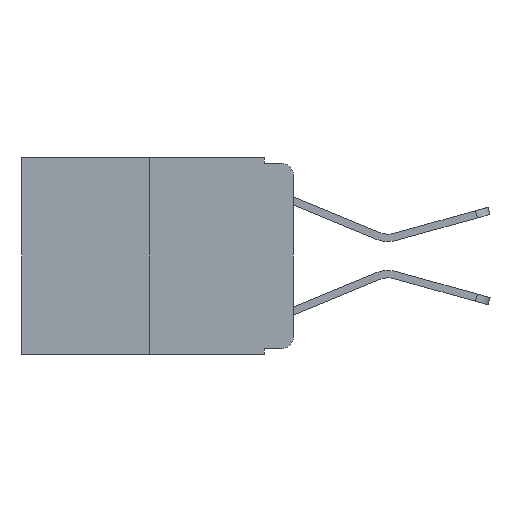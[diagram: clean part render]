
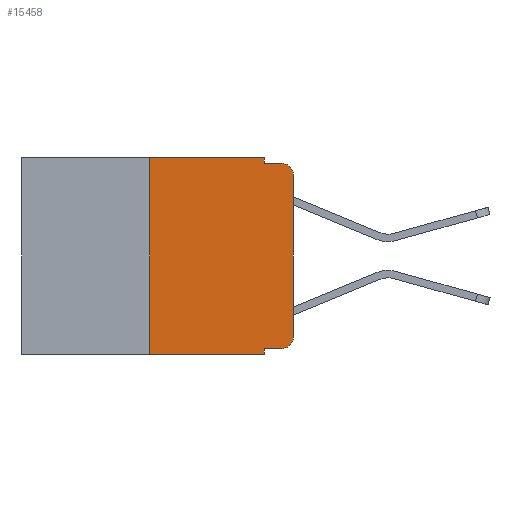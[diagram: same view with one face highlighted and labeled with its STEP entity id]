
A CAD part, left-side view. The second image highlights one B-rep face of the part: STEP entity #15458.
In plain terms, the highlighted planar face has unit normal (-1, 0, 0).
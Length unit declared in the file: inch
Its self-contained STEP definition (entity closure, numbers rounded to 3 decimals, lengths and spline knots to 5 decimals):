
#88 = CARTESIAN_POINT ( 'NONE',  ( 0., 0.051, -0.333 ) ) ;
#329 = CARTESIAN_POINT ( 'NONE',  ( 0., 0.051, -0.343 ) ) ;
#395 = FACE_OUTER_BOUND ( 'NONE', #11615, .T. ) ;
#422 = EDGE_CURVE ( 'NONE', #13965, #13686, #7644, .T. ) ;
#503 = DIRECTION ( 'NONE',  ( 0., 0., -1. ) ) ;
#634 = CARTESIAN_POINT ( 'NONE',  ( 0., 0.02, -0.03 ) ) ;
#659 = DIRECTION ( 'NONE',  ( 1., 0., 0. ) ) ;
#1108 = LINE ( 'NONE', #88, #8087 ) ;
#1526 = EDGE_CURVE ( 'NONE', #9423, #16759, #16364, .T. ) ;
#2062 = EDGE_CURVE ( 'NONE', #16759, #19306, #13859, .T. ) ;
#2522 = DIRECTION ( 'NONE',  ( 0., 0., -1. ) ) ;
#2666 = CARTESIAN_POINT ( 'NONE',  ( 0., 0.051, 0. ) ) ;
#3012 = EDGE_CURVE ( 'NONE', #3076, #13375, #11071, .T. ) ;
#3076 = VERTEX_POINT ( 'NONE', #5840 ) ;
#3400 = ORIENTED_EDGE ( 'NONE', *, *, #2062, .T. ) ;
#3526 = DIRECTION ( 'NONE',  ( 0., 0., 1. ) ) ;
#3726 = CARTESIAN_POINT ( 'NONE',  ( 0., 0., -0.313 ) ) ;
#3765 = CARTESIAN_POINT ( 'NONE',  ( 0., 0.25, 0. ) ) ;
#3791 = VECTOR ( 'NONE', #12204, 39.37008 ) ;
#4184 = VERTEX_POINT ( 'NONE', #16595 ) ;
#4256 = VERTEX_POINT ( 'NONE', #19798 ) ;
#4436 = CARTESIAN_POINT ( 'NONE',  ( 0., 0.473, -0.343 ) ) ;
#4549 = ORIENTED_EDGE ( 'NONE', *, *, #18521, .T. ) ;
#4565 = VECTOR ( 'NONE', #5202, 39.37008 ) ;
#4769 = LINE ( 'NONE', #18748, #3791 ) ;
#5177 = LINE ( 'NONE', #3765, #5943 ) ;
#5202 = DIRECTION ( 'NONE',  ( 0., -1., 0. ) ) ;
#5239 = PLANE ( 'NONE',  #6532 ) ;
#5347 = AXIS2_PLACEMENT_3D ( 'NONE', #20243, #10713, #20041 ) ;
#5450 = CARTESIAN_POINT ( 'NONE',  ( 0., 0.473, 0. ) ) ;
#5803 = CARTESIAN_POINT ( 'NONE',  ( 0., 0.051, -0.01 ) ) ;
#5840 = CARTESIAN_POINT ( 'NONE',  ( 0., 0.051, -0.333 ) ) ;
#5873 = VECTOR ( 'NONE', #3526, 39.37008 ) ;
#5907 = VECTOR ( 'NONE', #10166, 39.37008 ) ;
#5943 = VECTOR ( 'NONE', #16184, 39.37008 ) ;
#6349 = CARTESIAN_POINT ( 'NONE',  ( 0., 0.02, -0.01 ) ) ;
#6532 = AXIS2_PLACEMENT_3D ( 'NONE', #5450, #659, #6918 ) ;
#6845 = CARTESIAN_POINT ( 'NONE',  ( 0., 0.25, -0.343 ) ) ;
#6918 = DIRECTION ( 'NONE',  ( 0., 0., -1. ) ) ;
#7361 = LINE ( 'NONE', #4436, #14597 ) ;
#7644 = LINE ( 'NONE', #14907, #5907 ) ;
#7840 = VECTOR ( 'NONE', #2522, 39.37008 ) ;
#7985 = ORIENTED_EDGE ( 'NONE', *, *, #3012, .F. ) ;
#8087 = VECTOR ( 'NONE', #8300, 39.37008 ) ;
#8300 = DIRECTION ( 'NONE',  ( 0., -1., 0. ) ) ;
#8839 = CARTESIAN_POINT ( 'NONE',  ( 0., 0.473, 0. ) ) ;
#9423 = VERTEX_POINT ( 'NONE', #3726 ) ;
#10131 = ORIENTED_EDGE ( 'NONE', *, *, #16342, .F. ) ;
#10166 = DIRECTION ( 'NONE',  ( 0., 0., -1. ) ) ;
#10457 = ORIENTED_EDGE ( 'NONE', *, *, #15844, .T. ) ;
#10713 = DIRECTION ( 'NONE',  ( -1., 0., 0. ) ) ;
#10986 = EDGE_CURVE ( 'NONE', #13686, #19306, #4769, .T. ) ;
#11071 = LINE ( 'NONE', #2666, #7840 ) ;
#11073 = CARTESIAN_POINT ( 'NONE',  ( 0., 0., -0.03 ) ) ;
#11615 = EDGE_LOOP ( 'NONE', ( #16385, #3400, #16443, #11709, #16526, #10131, #4549, #7985, #10457, #14700 ) ) ;
#11709 = ORIENTED_EDGE ( 'NONE', *, *, #422, .F. ) ;
#12204 = DIRECTION ( 'NONE',  ( 0., -1., 0. ) ) ;
#12317 = LINE ( 'NONE', #8839, #4565 ) ;
#13375 = VERTEX_POINT ( 'NONE', #329 ) ;
#13686 = VERTEX_POINT ( 'NONE', #5803 ) ;
#13859 = CIRCLE ( 'NONE', #18254, 0.02 ) ;
#13965 = VERTEX_POINT ( 'NONE', #19108 ) ;
#14597 = VECTOR ( 'NONE', #17402, 39.37008 ) ;
#14700 = ORIENTED_EDGE ( 'NONE', *, *, #20493, .T. ) ;
#14907 = CARTESIAN_POINT ( 'NONE',  ( 0., 0.051, 0. ) ) ;
#15458 = ADVANCED_FACE ( 'NONE', ( #395 ), #5239, .F. ) ;
#15539 = VERTEX_POINT ( 'NONE', #6845 ) ;
#15844 = EDGE_CURVE ( 'NONE', #3076, #4256, #1108, .T. ) ;
#16184 = DIRECTION ( 'NONE',  ( 0., 0., 1. ) ) ;
#16342 = EDGE_CURVE ( 'NONE', #15539, #4184, #5177, .T. ) ;
#16364 = LINE ( 'NONE', #17872, #5873 ) ;
#16385 = ORIENTED_EDGE ( 'NONE', *, *, #1526, .T. ) ;
#16443 = ORIENTED_EDGE ( 'NONE', *, *, #10986, .F. ) ;
#16526 = ORIENTED_EDGE ( 'NONE', *, *, #20587, .F. ) ;
#16595 = CARTESIAN_POINT ( 'NONE',  ( 0., 0.25, 0. ) ) ;
#16759 = VERTEX_POINT ( 'NONE', #11073 ) ;
#17402 = DIRECTION ( 'NONE',  ( 0., -1., 0. ) ) ;
#17872 = CARTESIAN_POINT ( 'NONE',  ( 0., 0., 0. ) ) ;
#17914 = DIRECTION ( 'NONE',  ( -1., 0., 0. ) ) ;
#18254 = AXIS2_PLACEMENT_3D ( 'NONE', #634, #17914, #503 ) ;
#18521 = EDGE_CURVE ( 'NONE', #15539, #13375, #7361, .T. ) ;
#18748 = CARTESIAN_POINT ( 'NONE',  ( 0., 0.051, -0.01 ) ) ;
#19108 = CARTESIAN_POINT ( 'NONE',  ( 0., 0.051, 0. ) ) ;
#19302 = CIRCLE ( 'NONE', #5347, 0.02 ) ;
#19306 = VERTEX_POINT ( 'NONE', #6349 ) ;
#19798 = CARTESIAN_POINT ( 'NONE',  ( 0., 0.02, -0.333 ) ) ;
#20041 = DIRECTION ( 'NONE',  ( 0., 0., -1. ) ) ;
#20243 = CARTESIAN_POINT ( 'NONE',  ( 0., 0.02, -0.313 ) ) ;
#20493 = EDGE_CURVE ( 'NONE', #4256, #9423, #19302, .T. ) ;
#20587 = EDGE_CURVE ( 'NONE', #4184, #13965, #12317, .T. ) ;
